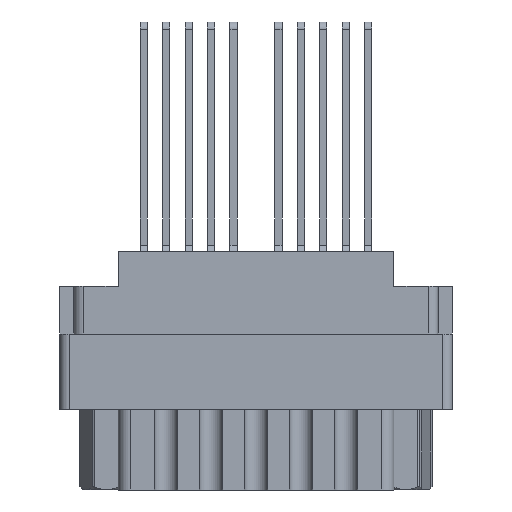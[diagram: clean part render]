
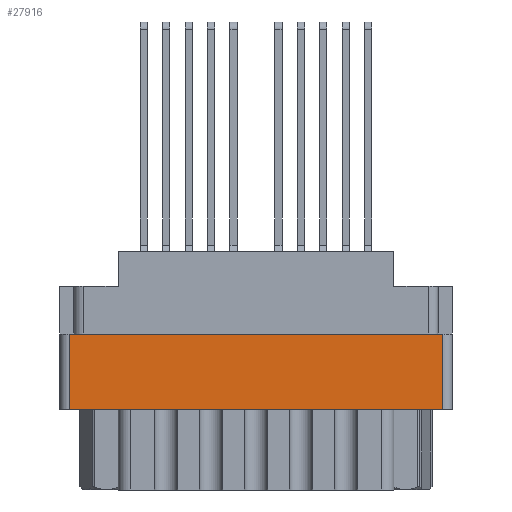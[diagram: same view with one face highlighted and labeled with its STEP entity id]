
A CAD part, front view. The second image highlights one B-rep face of the part: STEP entity #27916.
In plain terms, the highlighted planar face has unit normal (0, -1, 0).
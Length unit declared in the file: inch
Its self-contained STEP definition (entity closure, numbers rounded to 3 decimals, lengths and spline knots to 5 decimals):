
#2151 = LINE ( 'NONE', #29400, #22336 ) ;
#2879 = CARTESIAN_POINT ( 'NONE',  ( 0.624, -0.343, -0.277 ) ) ;
#3567 = EDGE_LOOP ( 'NONE', ( #19651, #23131, #30922, #32837 ) ) ;
#3994 = LINE ( 'NONE', #28439, #35813 ) ;
#5600 = DIRECTION ( 'NONE',  ( 1., 0., 0. ) ) ;
#5917 = EDGE_CURVE ( 'NONE', #16595, #30265, #9853, .T. ) ;
#8510 = PLANE ( 'NONE',  #11698 ) ;
#9631 = CARTESIAN_POINT ( 'NONE',  ( -0.624, -0.343, -0.529 ) ) ;
#9853 = LINE ( 'NONE', #25220, #21090 ) ;
#10635 = LINE ( 'NONE', #27054, #24086 ) ;
#11698 = AXIS2_PLACEMENT_3D ( 'NONE', #11866, #34590, #23290 ) ;
#11866 = CARTESIAN_POINT ( 'NONE',  ( -0.656, -0.343, -0.798 ) ) ;
#12594 = DIRECTION ( 'NONE',  ( 0., 0., -1. ) ) ;
#12899 = CARTESIAN_POINT ( 'NONE',  ( -0.624, -0.343, -0.277 ) ) ;
#13107 = CARTESIAN_POINT ( 'NONE',  ( 0.624, -0.343, -0.529 ) ) ;
#15718 = VERTEX_POINT ( 'NONE', #12899 ) ;
#16245 = FACE_OUTER_BOUND ( 'NONE', #3567, .T. ) ;
#16595 = VERTEX_POINT ( 'NONE', #13107 ) ;
#19271 = VERTEX_POINT ( 'NONE', #2879 ) ;
#19651 = ORIENTED_EDGE ( 'NONE', *, *, #30443, .F. ) ;
#21090 = VECTOR ( 'NONE', #30957, 39.37008 ) ;
#21421 = DIRECTION ( 'NONE',  ( 0., 0., 1. ) ) ;
#22336 = VECTOR ( 'NONE', #12594, 39.37008 ) ;
#23131 = ORIENTED_EDGE ( 'NONE', *, *, #30699, .T. ) ;
#23290 = DIRECTION ( 'NONE',  ( 0., 0., -1. ) ) ;
#24086 = VECTOR ( 'NONE', #21421, 39.37008 ) ;
#25220 = CARTESIAN_POINT ( 'NONE',  ( 0., -0.343, -0.529 ) ) ;
#27054 = CARTESIAN_POINT ( 'NONE',  ( 0.624, -0.343, -0.798 ) ) ;
#27916 = ADVANCED_FACE ( 'NONE', ( #16245 ), #8510, .T. ) ;
#28439 = CARTESIAN_POINT ( 'NONE',  ( 0., -0.343, -0.277 ) ) ;
#29400 = CARTESIAN_POINT ( 'NONE',  ( -0.624, -0.343, -0.798 ) ) ;
#29779 = EDGE_CURVE ( 'NONE', #16595, #19271, #10635, .T. ) ;
#30265 = VERTEX_POINT ( 'NONE', #9631 ) ;
#30443 = EDGE_CURVE ( 'NONE', #15718, #19271, #3994, .T. ) ;
#30699 = EDGE_CURVE ( 'NONE', #15718, #30265, #2151, .T. ) ;
#30922 = ORIENTED_EDGE ( 'NONE', *, *, #5917, .F. ) ;
#30957 = DIRECTION ( 'NONE',  ( -1., 0., 0. ) ) ;
#32837 = ORIENTED_EDGE ( 'NONE', *, *, #29779, .T. ) ;
#34590 = DIRECTION ( 'NONE',  ( 0., -1., 0. ) ) ;
#35813 = VECTOR ( 'NONE', #5600, 39.37008 ) ;
